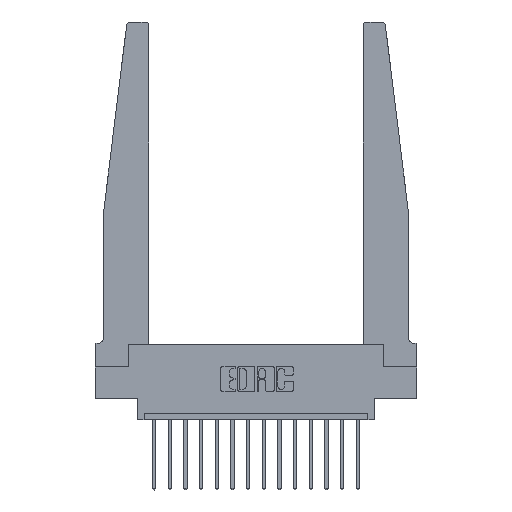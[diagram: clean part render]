
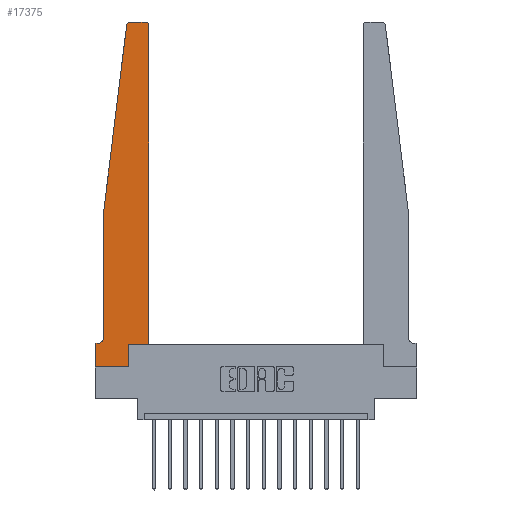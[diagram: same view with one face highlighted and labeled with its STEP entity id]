
A CAD part, top view. The second image highlights one B-rep face of the part: STEP entity #17375.
In plain terms, the highlighted planar face has unit normal (0, 0, 1).
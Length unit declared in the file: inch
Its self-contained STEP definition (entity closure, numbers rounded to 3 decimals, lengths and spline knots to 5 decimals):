
#127 = CARTESIAN_POINT ( 'NONE',  ( 0., 0.1875, 0.37 ) ) ;
#221 = DIRECTION ( 'NONE',  ( 1., 0., 0. ) ) ;
#563 = EDGE_CURVE ( 'NONE', #14151, #7877, #15455, .T. ) ;
#677 = CARTESIAN_POINT ( 'NONE',  ( 0.2605, 0., 0.37 ) ) ;
#789 = DIRECTION ( 'NONE',  ( 0., 1., 0. ) ) ;
#1194 = CARTESIAN_POINT ( 'NONE',  ( 0.065, 1.25, 0.37 ) ) ;
#1405 = CARTESIAN_POINT ( 'NONE',  ( 0.425, 0.18, 0.37 ) ) ;
#1449 = CARTESIAN_POINT ( 'NONE',  ( 0., 0., 0.37 ) ) ;
#1507 = ORIENTED_EDGE ( 'NONE', *, *, #16957, .T. ) ;
#1555 = LINE ( 'NONE', #10941, #17093 ) ;
#1599 = LINE ( 'NONE', #2736, #13784 ) ;
#1927 = VECTOR ( 'NONE', #12403, 39.37008 ) ;
#2016 = VECTOR ( 'NONE', #6484, 39.37008 ) ;
#2188 = VERTEX_POINT ( 'NONE', #10455 ) ;
#2615 = DIRECTION ( 'NONE',  ( -0.122, -0.992, 0. ) ) ;
#2736 = CARTESIAN_POINT ( 'NONE',  ( 0., 0., 0.37 ) ) ;
#2852 = EDGE_CURVE ( 'NONE', #10118, #15926, #14721, .T. ) ;
#2976 = ORIENTED_EDGE ( 'NONE', *, *, #9354, .T. ) ;
#2993 = AXIS2_PLACEMENT_3D ( 'NONE', #11165, #5660, #221 ) ;
#3021 = DIRECTION ( 'NONE',  ( 0., 1., 0. ) ) ;
#3346 = EDGE_CURVE ( 'NONE', #6054, #11919, #12440, .T. ) ;
#3467 = CARTESIAN_POINT ( 'NONE',  ( 0.065, 0.2375, 0.37 ) ) ;
#3602 = CARTESIAN_POINT ( 'NONE',  ( 0.2605, 0.18, 0.37 ) ) ;
#3703 = LINE ( 'NONE', #6418, #2016 ) ;
#3773 = VECTOR ( 'NONE', #5550, 39.37008 ) ;
#3781 = CARTESIAN_POINT ( 'NONE',  ( 0.425, 2.72, 0.37 ) ) ;
#4054 = CARTESIAN_POINT ( 'NONE',  ( 0.065, 1.25, 0.37 ) ) ;
#4198 = CARTESIAN_POINT ( 'NONE',  ( 0.395, 2.75, 0.37 ) ) ;
#4217 = ORIENTED_EDGE ( 'NONE', *, *, #2852, .T. ) ;
#4384 = CARTESIAN_POINT ( 'NONE',  ( 0.065, 1.25, 0.37 ) ) ;
#4479 = EDGE_LOOP ( 'NONE', ( #17268, #6583, #13145, #4217, #1507, #11169, #12974, #16435, #10535, #2976, #8183, #6569 ) ) ;
#4507 = CARTESIAN_POINT ( 'NONE',  ( 0.27653, 2.75, 0.37 ) ) ;
#4509 = EDGE_CURVE ( 'NONE', #12823, #10118, #14003, .T. ) ;
#4721 = CARTESIAN_POINT ( 'NONE',  ( 0.27653, 2.72, 0.37 ) ) ;
#5206 = DIRECTION ( 'NONE',  ( -1., 0., 0. ) ) ;
#5254 = VERTEX_POINT ( 'NONE', #1405 ) ;
#5390 = VERTEX_POINT ( 'NONE', #677 ) ;
#5550 = DIRECTION ( 'NONE',  ( -1., 0., 0. ) ) ;
#5660 = DIRECTION ( 'NONE',  ( 0., 0., 1. ) ) ;
#5806 = DIRECTION ( 'NONE',  ( 0., -1., 0. ) ) ;
#5902 = VECTOR ( 'NONE', #3021, 39.37008 ) ;
#6054 = VERTEX_POINT ( 'NONE', #127 ) ;
#6185 = DIRECTION ( 'NONE',  ( 0., 0., 1. ) ) ;
#6304 = FACE_OUTER_BOUND ( 'NONE', #4479, .T. ) ;
#6322 = EDGE_CURVE ( 'NONE', #5390, #9790, #15297, .T. ) ;
#6418 = CARTESIAN_POINT ( 'NONE',  ( 0.425, 0.18, 0.37 ) ) ;
#6484 = DIRECTION ( 'NONE',  ( 1., 0., 0. ) ) ;
#6489 = CARTESIAN_POINT ( 'NONE',  ( 0.015, 0.2375, 0.37 ) ) ;
#6569 = ORIENTED_EDGE ( 'NONE', *, *, #563, .T. ) ;
#6583 = ORIENTED_EDGE ( 'NONE', *, *, #12124, .T. ) ;
#6875 = CARTESIAN_POINT ( 'NONE',  ( 0.2605, 0.18, 0.37 ) ) ;
#7446 = DIRECTION ( 'NONE',  ( 1., 0., 0. ) ) ;
#7618 = CARTESIAN_POINT ( 'NONE',  ( 0., 0.1875, 0.37 ) ) ;
#7659 = EDGE_CURVE ( 'NONE', #7877, #10231, #11138, .T. ) ;
#7716 = DIRECTION ( 'NONE',  ( -1., 0., 0. ) ) ;
#7771 = VECTOR ( 'NONE', #5806, 39.37008 ) ;
#7877 = VERTEX_POINT ( 'NONE', #4198 ) ;
#8183 = ORIENTED_EDGE ( 'NONE', *, *, #11171, .T. ) ;
#8489 = CARTESIAN_POINT ( 'NONE',  ( 0., 0., 0.37 ) ) ;
#8964 = DIRECTION ( 'NONE',  ( 0., 0., 1. ) ) ;
#9354 = EDGE_CURVE ( 'NONE', #9790, #5254, #3703, .T. ) ;
#9790 = VERTEX_POINT ( 'NONE', #3602 ) ;
#10118 = VERTEX_POINT ( 'NONE', #4054 ) ;
#10231 = VERTEX_POINT ( 'NONE', #4507 ) ;
#10275 = PLANE ( 'NONE',  #13140 ) ;
#10455 = CARTESIAN_POINT ( 'NONE',  ( 0.015, 0.1875, 0.37 ) ) ;
#10493 = EDGE_CURVE ( 'NONE', #2188, #6054, #1555, .T. ) ;
#10535 = ORIENTED_EDGE ( 'NONE', *, *, #6322, .T. ) ;
#10557 = DIRECTION ( 'NONE',  ( 0., 0., -1. ) ) ;
#10941 = CARTESIAN_POINT ( 'NONE',  ( 0.065, 0.1875, 0.37 ) ) ;
#11078 = VECTOR ( 'NONE', #2615, 39.37008 ) ;
#11138 = LINE ( 'NONE', #12138, #3773 ) ;
#11165 = CARTESIAN_POINT ( 'NONE',  ( 0.395, 2.72, 0.37 ) ) ;
#11169 = ORIENTED_EDGE ( 'NONE', *, *, #10493, .T. ) ;
#11171 = EDGE_CURVE ( 'NONE', #5254, #14151, #17053, .T. ) ;
#11534 = CARTESIAN_POINT ( 'NONE',  ( 0.425, 0.18, 0.37 ) ) ;
#11919 = VERTEX_POINT ( 'NONE', #8489 ) ;
#11977 = AXIS2_PLACEMENT_3D ( 'NONE', #4721, #6185, #7446 ) ;
#12025 = AXIS2_PLACEMENT_3D ( 'NONE', #6489, #10557, #5206 ) ;
#12124 = EDGE_CURVE ( 'NONE', #10231, #12823, #13495, .T. ) ;
#12138 = CARTESIAN_POINT ( 'NONE',  ( 0.25, 2.75, 0.37 ) ) ;
#12403 = DIRECTION ( 'NONE',  ( 0., -1., 0. ) ) ;
#12440 = LINE ( 'NONE', #1449, #1927 ) ;
#12823 = VERTEX_POINT ( 'NONE', #15931 ) ;
#12974 = ORIENTED_EDGE ( 'NONE', *, *, #3346, .T. ) ;
#13140 = AXIS2_PLACEMENT_3D ( 'NONE', #7618, #8964, #14711 ) ;
#13145 = ORIENTED_EDGE ( 'NONE', *, *, #4509, .T. ) ;
#13495 = CIRCLE ( 'NONE', #11977, 0.03 ) ;
#13512 = VECTOR ( 'NONE', #789, 39.37008 ) ;
#13784 = VECTOR ( 'NONE', #16034, 39.37008 ) ;
#14003 = LINE ( 'NONE', #1194, #11078 ) ;
#14151 = VERTEX_POINT ( 'NONE', #3781 ) ;
#14711 = DIRECTION ( 'NONE',  ( 1., 0., 0. ) ) ;
#14721 = LINE ( 'NONE', #4384, #7771 ) ;
#15243 = EDGE_CURVE ( 'NONE', #11919, #5390, #1599, .T. ) ;
#15297 = LINE ( 'NONE', #6875, #5902 ) ;
#15455 = CIRCLE ( 'NONE', #2993, 0.03 ) ;
#15792 = CIRCLE ( 'NONE', #12025, 0.05 ) ;
#15926 = VERTEX_POINT ( 'NONE', #3467 ) ;
#15931 = CARTESIAN_POINT ( 'NONE',  ( 0.24675, 2.72367, 0.37 ) ) ;
#16034 = DIRECTION ( 'NONE',  ( 1., 0., 0. ) ) ;
#16435 = ORIENTED_EDGE ( 'NONE', *, *, #15243, .T. ) ;
#16957 = EDGE_CURVE ( 'NONE', #15926, #2188, #15792, .T. ) ;
#17053 = LINE ( 'NONE', #11534, #13512 ) ;
#17093 = VECTOR ( 'NONE', #7716, 39.37008 ) ;
#17268 = ORIENTED_EDGE ( 'NONE', *, *, #7659, .T. ) ;
#17375 = ADVANCED_FACE ( 'NONE', ( #6304 ), #10275, .T. ) ;
